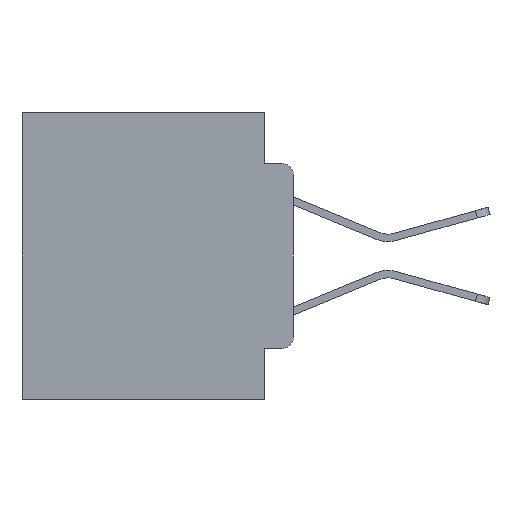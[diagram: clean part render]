
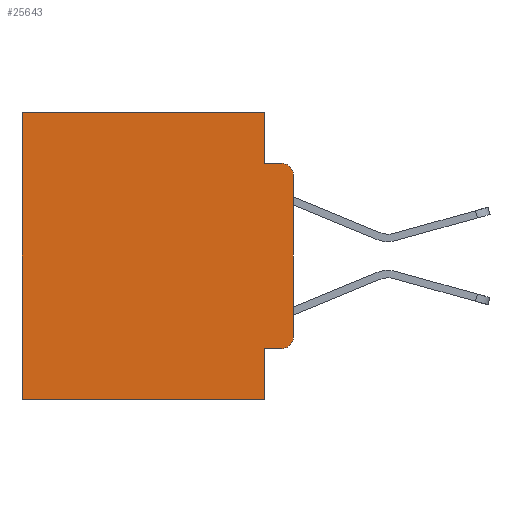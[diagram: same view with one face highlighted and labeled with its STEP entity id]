
A CAD part, left-side view. The second image highlights one B-rep face of the part: STEP entity #25643.
In plain terms, the highlighted planar face has unit normal (-1, 0, 0).
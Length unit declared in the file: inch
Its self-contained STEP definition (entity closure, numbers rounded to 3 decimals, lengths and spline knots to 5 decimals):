
#69 = VERTEX_POINT ( 'NONE', #13389 ) ;
#118 = CARTESIAN_POINT ( 'NONE',  ( 0.298, 0., -0.3915 ) ) ;
#486 = DIRECTION ( 'NONE',  ( 0., 1., 0. ) ) ;
#487 = VERTEX_POINT ( 'NONE', #21042 ) ;
#1860 = DIRECTION ( 'NONE',  ( 0., 0., -1. ) ) ;
#2048 = CARTESIAN_POINT ( 'NONE',  ( 0.298, 0.051, -0.5 ) ) ;
#2066 = ORIENTED_EDGE ( 'NONE', *, *, #22773, .F. ) ;
#2120 = VERTEX_POINT ( 'NONE', #13112 ) ;
#2478 = AXIS2_PLACEMENT_3D ( 'NONE', #22453, #10357, #24449 ) ;
#2550 = CARTESIAN_POINT ( 'NONE',  ( 0.298, 0.473, 0. ) ) ;
#3042 = VECTOR ( 'NONE', #21638, 39.37008 ) ;
#4296 = EDGE_CURVE ( 'NONE', #14362, #19393, #7216, .T. ) ;
#4580 = VERTEX_POINT ( 'NONE', #20678 ) ;
#5435 = CARTESIAN_POINT ( 'NONE',  ( 0.298, 0.051, 0. ) ) ;
#5796 = EDGE_CURVE ( 'NONE', #25730, #14239, #8774, .T. ) ;
#6483 = DIRECTION ( 'NONE',  ( 1., 0., 0. ) ) ;
#6531 = VECTOR ( 'NONE', #13852, 39.37008 ) ;
#6553 = ORIENTED_EDGE ( 'NONE', *, *, #26569, .T. ) ;
#6789 = VECTOR ( 'NONE', #18392, 39.37008 ) ;
#7023 = DIRECTION ( 'NONE',  ( 0., -1., 0. ) ) ;
#7074 = CARTESIAN_POINT ( 'NONE',  ( 0.298, 0., -0.5 ) ) ;
#7216 = LINE ( 'NONE', #5435, #6531 ) ;
#7261 = EDGE_CURVE ( 'NONE', #69, #487, #25126, .T. ) ;
#7576 = CIRCLE ( 'NONE', #2478, 0.02 ) ;
#8363 = CARTESIAN_POINT ( 'NONE',  ( 0.298, 0.02, -0.1085 ) ) ;
#8774 = LINE ( 'NONE', #16409, #6789 ) ;
#8899 = CARTESIAN_POINT ( 'NONE',  ( 0.298, 0., -0.1085 ) ) ;
#9309 = AXIS2_PLACEMENT_3D ( 'NONE', #18733, #6483, #20766 ) ;
#9483 = VECTOR ( 'NONE', #21549, 39.37008 ) ;
#10357 = DIRECTION ( 'NONE',  ( -1., 0., 0. ) ) ;
#10418 = EDGE_CURVE ( 'NONE', #17217, #14239, #7576, .T. ) ;
#10456 = DIRECTION ( 'NONE',  ( 0., 0., -1. ) ) ;
#10825 = ORIENTED_EDGE ( 'NONE', *, *, #10418, .T. ) ;
#11922 = LINE ( 'NONE', #21258, #12551 ) ;
#12314 = CIRCLE ( 'NONE', #21010, 0.02 ) ;
#12551 = VECTOR ( 'NONE', #7023, 39.37008 ) ;
#13112 = CARTESIAN_POINT ( 'NONE',  ( 0.298, 0.051, -0.0885 ) ) ;
#13389 = CARTESIAN_POINT ( 'NONE',  ( 0.298, 0.473, 0. ) ) ;
#13496 = VERTEX_POINT ( 'NONE', #14647 ) ;
#13836 = VECTOR ( 'NONE', #15201, 39.37008 ) ;
#13852 = DIRECTION ( 'NONE',  ( 0., 0., -1. ) ) ;
#14016 = ORIENTED_EDGE ( 'NONE', *, *, #24055, .T. ) ;
#14239 = VERTEX_POINT ( 'NONE', #118 ) ;
#14339 = EDGE_CURVE ( 'NONE', #19393, #487, #20878, .T. ) ;
#14362 = VERTEX_POINT ( 'NONE', #23343 ) ;
#14520 = FACE_OUTER_BOUND ( 'NONE', #15354, .T. ) ;
#14647 = CARTESIAN_POINT ( 'NONE',  ( 0.298, 0.02, -0.0885 ) ) ;
#14934 = LINE ( 'NONE', #25563, #3042 ) ;
#15201 = DIRECTION ( 'NONE',  ( 0., 0., -1. ) ) ;
#15354 = EDGE_LOOP ( 'NONE', ( #16539, #24686, #20608, #2066, #14016, #17471, #23469, #16842, #6553, #10825 ) ) ;
#15719 = CARTESIAN_POINT ( 'NONE',  ( 0.298, 0.02, -0.4115 ) ) ;
#16031 = EDGE_CURVE ( 'NONE', #25730, #13496, #12314, .T. ) ;
#16409 = CARTESIAN_POINT ( 'NONE',  ( 0.298, 0., 0. ) ) ;
#16539 = ORIENTED_EDGE ( 'NONE', *, *, #5796, .F. ) ;
#16842 = ORIENTED_EDGE ( 'NONE', *, *, #4296, .F. ) ;
#17217 = VERTEX_POINT ( 'NONE', #15719 ) ;
#17471 = ORIENTED_EDGE ( 'NONE', *, *, #7261, .T. ) ;
#18392 = DIRECTION ( 'NONE',  ( 0., 0., -1. ) ) ;
#18733 = CARTESIAN_POINT ( 'NONE',  ( 0.298, 0., 0. ) ) ;
#19326 = VECTOR ( 'NONE', #1860, 39.37008 ) ;
#19393 = VERTEX_POINT ( 'NONE', #2048 ) ;
#19522 = CARTESIAN_POINT ( 'NONE',  ( 0.298, 0., 0. ) ) ;
#19956 = LINE ( 'NONE', #26535, #19326 ) ;
#20245 = LINE ( 'NONE', #19522, #9483 ) ;
#20608 = ORIENTED_EDGE ( 'NONE', *, *, #24090, .F. ) ;
#20678 = CARTESIAN_POINT ( 'NONE',  ( 0.298, 0.051, 0. ) ) ;
#20766 = DIRECTION ( 'NONE',  ( 0., 0., -1. ) ) ;
#20878 = LINE ( 'NONE', #7074, #25576 ) ;
#21010 = AXIS2_PLACEMENT_3D ( 'NONE', #8363, #22550, #10456 ) ;
#21042 = CARTESIAN_POINT ( 'NONE',  ( 0.298, 0.473, -0.5 ) ) ;
#21258 = CARTESIAN_POINT ( 'NONE',  ( 0.298, 0.051, -0.4115 ) ) ;
#21549 = DIRECTION ( 'NONE',  ( 0., 1., 0. ) ) ;
#21638 = DIRECTION ( 'NONE',  ( 0., -1., 0. ) ) ;
#22453 = CARTESIAN_POINT ( 'NONE',  ( 0.298, 0.02, -0.3915 ) ) ;
#22550 = DIRECTION ( 'NONE',  ( -1., 0., 0. ) ) ;
#22773 = EDGE_CURVE ( 'NONE', #4580, #2120, #19956, .T. ) ;
#23343 = CARTESIAN_POINT ( 'NONE',  ( 0.298, 0.051, -0.4115 ) ) ;
#23469 = ORIENTED_EDGE ( 'NONE', *, *, #14339, .F. ) ;
#24055 = EDGE_CURVE ( 'NONE', #4580, #69, #20245, .T. ) ;
#24090 = EDGE_CURVE ( 'NONE', #2120, #13496, #14934, .T. ) ;
#24449 = DIRECTION ( 'NONE',  ( 0., 0., -1. ) ) ;
#24686 = ORIENTED_EDGE ( 'NONE', *, *, #16031, .T. ) ;
#25126 = LINE ( 'NONE', #2550, #13836 ) ;
#25563 = CARTESIAN_POINT ( 'NONE',  ( 0.298, 0.051, -0.0885 ) ) ;
#25576 = VECTOR ( 'NONE', #486, 39.37008 ) ;
#25643 = ADVANCED_FACE ( 'NONE', ( #14520 ), #26699, .F. ) ;
#25730 = VERTEX_POINT ( 'NONE', #8899 ) ;
#26535 = CARTESIAN_POINT ( 'NONE',  ( 0.298, 0.051, 0. ) ) ;
#26569 = EDGE_CURVE ( 'NONE', #14362, #17217, #11922, .T. ) ;
#26699 = PLANE ( 'NONE',  #9309 ) ;
